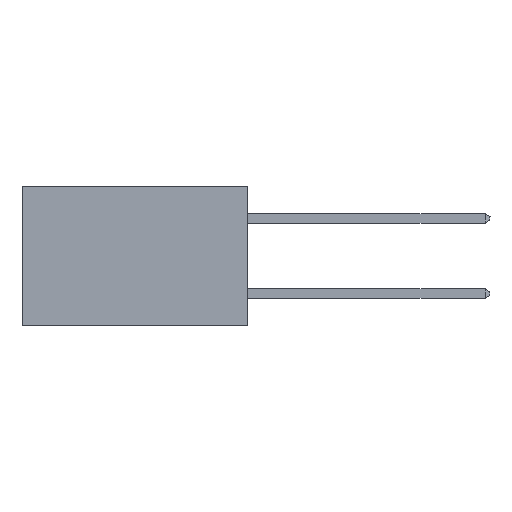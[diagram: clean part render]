
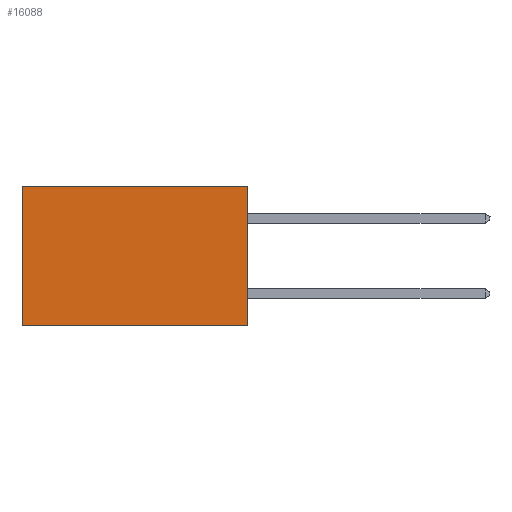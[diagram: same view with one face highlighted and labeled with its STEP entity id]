
A CAD part, left-side view. The second image highlights one B-rep face of the part: STEP entity #16088.
In plain terms, the highlighted planar face has unit normal (-1, 0, 0).
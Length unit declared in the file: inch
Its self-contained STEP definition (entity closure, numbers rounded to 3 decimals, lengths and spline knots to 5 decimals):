
#477 = ORIENTED_EDGE ( 'NONE', *, *, #12748, .F. ) ;
#704 = DIRECTION ( 'NONE',  ( 0., 0., -1. ) ) ;
#1525 = DIRECTION ( 'NONE',  ( 0., 0., -1. ) ) ;
#1781 = VECTOR ( 'NONE', #704, 39.37008 ) ;
#1910 = LINE ( 'NONE', #12582, #1781 ) ;
#2804 = EDGE_CURVE ( 'NONE', #11593, #12432, #15976, .T. ) ;
#2947 = DIRECTION ( 'NONE',  ( 1., 0., 0. ) ) ;
#3662 = VERTEX_POINT ( 'NONE', #8793 ) ;
#3965 = DIRECTION ( 'NONE',  ( 0., 1., 0. ) ) ;
#4039 = CARTESIAN_POINT ( 'NONE',  ( 0.2615, 0., -0.37 ) ) ;
#4374 = AXIS2_PLACEMENT_3D ( 'NONE', #5804, #2947, #6833 ) ;
#5804 = CARTESIAN_POINT ( 'NONE',  ( 0.2615, 0., -0.37 ) ) ;
#6469 = CARTESIAN_POINT ( 'NONE',  ( 0.2615, 0., 0. ) ) ;
#6696 = LINE ( 'NONE', #14517, #10562 ) ;
#6833 = DIRECTION ( 'NONE',  ( 0., 0., -1. ) ) ;
#6996 = EDGE_CURVE ( 'NONE', #8313, #3662, #7671, .T. ) ;
#7671 = LINE ( 'NONE', #6469, #14865 ) ;
#8297 = ORIENTED_EDGE ( 'NONE', *, *, #6996, .T. ) ;
#8313 = VERTEX_POINT ( 'NONE', #9766 ) ;
#8346 = VECTOR ( 'NONE', #15804, 39.37008 ) ;
#8793 = CARTESIAN_POINT ( 'NONE',  ( 0.2615, 0.6, 0. ) ) ;
#9766 = CARTESIAN_POINT ( 'NONE',  ( 0.2615, 0., 0. ) ) ;
#10552 = CARTESIAN_POINT ( 'NONE',  ( 0.2615, 0., -0.37 ) ) ;
#10562 = VECTOR ( 'NONE', #1525, 39.37008 ) ;
#11593 = VERTEX_POINT ( 'NONE', #4039 ) ;
#12097 = EDGE_CURVE ( 'NONE', #3662, #12432, #6696, .T. ) ;
#12432 = VERTEX_POINT ( 'NONE', #14004 ) ;
#12582 = CARTESIAN_POINT ( 'NONE',  ( 0.2615, 0., -0.37 ) ) ;
#12748 = EDGE_CURVE ( 'NONE', #8313, #11593, #1910, .T. ) ;
#13655 = EDGE_LOOP ( 'NONE', ( #14118, #15279, #477, #8297 ) ) ;
#13711 = PLANE ( 'NONE',  #4374 ) ;
#14004 = CARTESIAN_POINT ( 'NONE',  ( 0.2615, 0.6, -0.37 ) ) ;
#14118 = ORIENTED_EDGE ( 'NONE', *, *, #12097, .T. ) ;
#14517 = CARTESIAN_POINT ( 'NONE',  ( 0.2615, 0.6, -0.37 ) ) ;
#14865 = VECTOR ( 'NONE', #3965, 39.37008 ) ;
#14911 = FACE_OUTER_BOUND ( 'NONE', #13655, .T. ) ;
#15279 = ORIENTED_EDGE ( 'NONE', *, *, #2804, .F. ) ;
#15804 = DIRECTION ( 'NONE',  ( 0., 1., 0. ) ) ;
#15976 = LINE ( 'NONE', #10552, #8346 ) ;
#16088 = ADVANCED_FACE ( 'NONE', ( #14911 ), #13711, .F. ) ;
